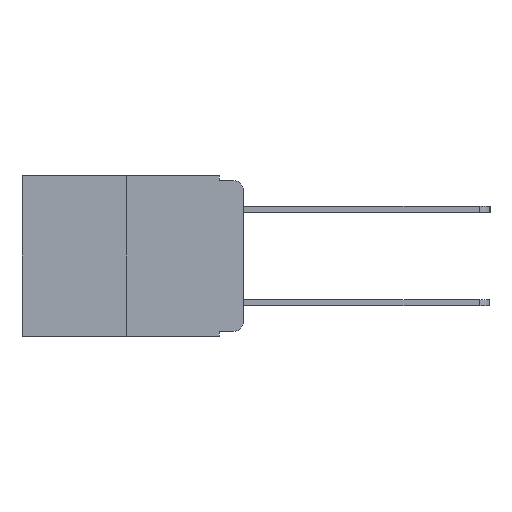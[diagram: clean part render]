
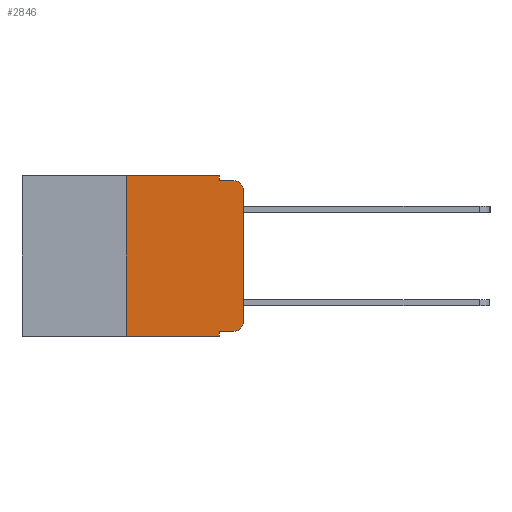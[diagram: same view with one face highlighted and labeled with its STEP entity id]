
A CAD part, left-side view. The second image highlights one B-rep face of the part: STEP entity #2846.
In plain terms, the highlighted planar face has unit normal (-1, 0, 0).
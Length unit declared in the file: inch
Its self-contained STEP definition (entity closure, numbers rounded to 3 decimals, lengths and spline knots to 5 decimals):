
#69 = VECTOR ( 'NONE', #1857, 39.37008 ) ;
#172 = ORIENTED_EDGE ( 'NONE', *, *, #1983, .T. ) ;
#245 = EDGE_CURVE ( 'NONE', #7105, #8514, #9768, .T. ) ;
#254 = VERTEX_POINT ( 'NONE', #8883 ) ;
#302 = VECTOR ( 'NONE', #4080, 39.37008 ) ;
#309 = LINE ( 'NONE', #8798, #2854 ) ;
#344 = LINE ( 'NONE', #7728, #7276 ) ;
#427 = VECTOR ( 'NONE', #4000, 39.37008 ) ;
#599 = CARTESIAN_POINT ( 'NONE',  ( 0., 0.02, -0.333 ) ) ;
#912 = VECTOR ( 'NONE', #9824, 39.37008 ) ;
#1275 = CARTESIAN_POINT ( 'NONE',  ( 0., 0.051, -0.01 ) ) ;
#1370 = VECTOR ( 'NONE', #10472, 39.37008 ) ;
#1659 = CARTESIAN_POINT ( 'NONE',  ( 0., 0., -0.313 ) ) ;
#1796 = ORIENTED_EDGE ( 'NONE', *, *, #4678, .F. ) ;
#1857 = DIRECTION ( 'NONE',  ( 0., -1., 0. ) ) ;
#1983 = EDGE_CURVE ( 'NONE', #8942, #3719, #309, .T. ) ;
#2089 = ORIENTED_EDGE ( 'NONE', *, *, #6801, .F. ) ;
#2423 = VERTEX_POINT ( 'NONE', #4504 ) ;
#2428 = DIRECTION ( 'NONE',  ( 0., 0., -1. ) ) ;
#2547 = VERTEX_POINT ( 'NONE', #1275 ) ;
#2597 = LINE ( 'NONE', #5532, #69 ) ;
#2846 = ADVANCED_FACE ( 'NONE', ( #10875 ), #7620, .F. ) ;
#2850 = LINE ( 'NONE', #8290, #302 ) ;
#2854 = VECTOR ( 'NONE', #9208, 39.37008 ) ;
#2979 = CARTESIAN_POINT ( 'NONE',  ( 0., 0., 0. ) ) ;
#2982 = LINE ( 'NONE', #9031, #427 ) ;
#3042 = VERTEX_POINT ( 'NONE', #4130 ) ;
#3467 = DIRECTION ( 'NONE',  ( 1., 0., 0. ) ) ;
#3538 = EDGE_LOOP ( 'NONE', ( #5278, #5554, #10093, #3756, #1796, #2089, #6858, #11052, #172, #9503 ) ) ;
#3609 = CARTESIAN_POINT ( 'NONE',  ( 0., 0.02, -0.03 ) ) ;
#3719 = VERTEX_POINT ( 'NONE', #599 ) ;
#3756 = ORIENTED_EDGE ( 'NONE', *, *, #8435, .F. ) ;
#4000 = DIRECTION ( 'NONE',  ( 0., 0., -1. ) ) ;
#4080 = DIRECTION ( 'NONE',  ( 0., 0., 1. ) ) ;
#4130 = CARTESIAN_POINT ( 'NONE',  ( 0., 0.051, 0. ) ) ;
#4283 = EDGE_CURVE ( 'NONE', #2547, #254, #2597, .T. ) ;
#4314 = AXIS2_PLACEMENT_3D ( 'NONE', #9403, #4437, #10166 ) ;
#4379 = EDGE_CURVE ( 'NONE', #2423, #8543, #6258, .T. ) ;
#4437 = DIRECTION ( 'NONE',  ( -1., 0., 0. ) ) ;
#4498 = DIRECTION ( 'NONE',  ( 0., 0., -1. ) ) ;
#4504 = CARTESIAN_POINT ( 'NONE',  ( 0., 0.25, -0.343 ) ) ;
#4620 = VECTOR ( 'NONE', #8789, 39.37008 ) ;
#4678 = EDGE_CURVE ( 'NONE', #5146, #3042, #344, .T. ) ;
#4735 = EDGE_CURVE ( 'NONE', #3719, #7105, #4762, .T. ) ;
#4762 = CIRCLE ( 'NONE', #4314, 0.02 ) ;
#5011 = CARTESIAN_POINT ( 'NONE',  ( 0., 0.25, 0. ) ) ;
#5103 = EDGE_CURVE ( 'NONE', #8942, #8543, #7771, .T. ) ;
#5146 = VERTEX_POINT ( 'NONE', #5011 ) ;
#5278 = ORIENTED_EDGE ( 'NONE', *, *, #245, .T. ) ;
#5477 = EDGE_CURVE ( 'NONE', #8514, #254, #10811, .T. ) ;
#5532 = CARTESIAN_POINT ( 'NONE',  ( 0., 0.051, -0.01 ) ) ;
#5554 = ORIENTED_EDGE ( 'NONE', *, *, #5477, .T. ) ;
#5598 = CARTESIAN_POINT ( 'NONE',  ( 0., 0.051, -0.333 ) ) ;
#6258 = LINE ( 'NONE', #9707, #1370 ) ;
#6801 = EDGE_CURVE ( 'NONE', #2423, #5146, #2850, .T. ) ;
#6858 = ORIENTED_EDGE ( 'NONE', *, *, #4379, .T. ) ;
#7051 = CARTESIAN_POINT ( 'NONE',  ( 0., 0.473, 0. ) ) ;
#7105 = VERTEX_POINT ( 'NONE', #1659 ) ;
#7276 = VECTOR ( 'NONE', #8530, 39.37008 ) ;
#7458 = AXIS2_PLACEMENT_3D ( 'NONE', #3609, #9457, #4498 ) ;
#7620 = PLANE ( 'NONE',  #7969 ) ;
#7728 = CARTESIAN_POINT ( 'NONE',  ( 0., 0.473, 0. ) ) ;
#7771 = LINE ( 'NONE', #9056, #912 ) ;
#7969 = AXIS2_PLACEMENT_3D ( 'NONE', #7051, #3467, #2428 ) ;
#8290 = CARTESIAN_POINT ( 'NONE',  ( 0., 0.25, 0. ) ) ;
#8435 = EDGE_CURVE ( 'NONE', #3042, #2547, #2982, .T. ) ;
#8514 = VERTEX_POINT ( 'NONE', #9101 ) ;
#8530 = DIRECTION ( 'NONE',  ( 0., -1., 0. ) ) ;
#8543 = VERTEX_POINT ( 'NONE', #10628 ) ;
#8789 = DIRECTION ( 'NONE',  ( 0., 0., 1. ) ) ;
#8798 = CARTESIAN_POINT ( 'NONE',  ( 0., 0.051, -0.333 ) ) ;
#8883 = CARTESIAN_POINT ( 'NONE',  ( 0., 0.02, -0.01 ) ) ;
#8942 = VERTEX_POINT ( 'NONE', #5598 ) ;
#9031 = CARTESIAN_POINT ( 'NONE',  ( 0., 0.051, 0. ) ) ;
#9056 = CARTESIAN_POINT ( 'NONE',  ( 0., 0.051, 0. ) ) ;
#9101 = CARTESIAN_POINT ( 'NONE',  ( 0., 0., -0.03 ) ) ;
#9208 = DIRECTION ( 'NONE',  ( 0., -1., 0. ) ) ;
#9403 = CARTESIAN_POINT ( 'NONE',  ( 0., 0.02, -0.313 ) ) ;
#9457 = DIRECTION ( 'NONE',  ( -1., 0., 0. ) ) ;
#9503 = ORIENTED_EDGE ( 'NONE', *, *, #4735, .T. ) ;
#9707 = CARTESIAN_POINT ( 'NONE',  ( 0., 0.473, -0.343 ) ) ;
#9768 = LINE ( 'NONE', #2979, #4620 ) ;
#9824 = DIRECTION ( 'NONE',  ( 0., 0., -1. ) ) ;
#10093 = ORIENTED_EDGE ( 'NONE', *, *, #4283, .F. ) ;
#10166 = DIRECTION ( 'NONE',  ( 0., 0., -1. ) ) ;
#10472 = DIRECTION ( 'NONE',  ( 0., -1., 0. ) ) ;
#10628 = CARTESIAN_POINT ( 'NONE',  ( 0., 0.051, -0.343 ) ) ;
#10811 = CIRCLE ( 'NONE', #7458, 0.02 ) ;
#10875 = FACE_OUTER_BOUND ( 'NONE', #3538, .T. ) ;
#11052 = ORIENTED_EDGE ( 'NONE', *, *, #5103, .F. ) ;
